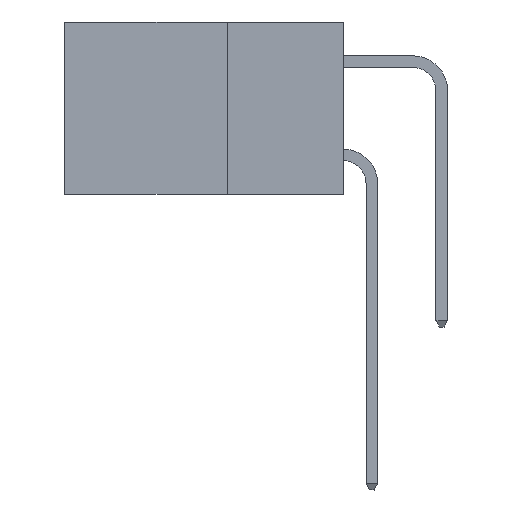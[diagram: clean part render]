
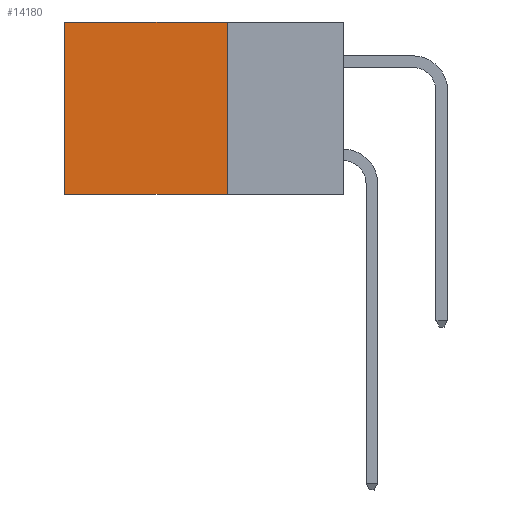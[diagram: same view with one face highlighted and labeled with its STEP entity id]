
A CAD part, left-side view. The second image highlights one B-rep face of the part: STEP entity #14180.
In plain terms, the highlighted planar face has unit normal (-1, 0, 0).
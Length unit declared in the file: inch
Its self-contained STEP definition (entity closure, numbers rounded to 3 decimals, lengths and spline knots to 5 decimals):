
#295 = ORIENTED_EDGE ( 'NONE', *, *, #18382, .F. ) ;
#797 = ORIENTED_EDGE ( 'NONE', *, *, #12884, .F. ) ;
#1860 = DIRECTION ( 'NONE',  ( 0., 1., 0. ) ) ;
#2047 = VECTOR ( 'NONE', #17260, 39.37008 ) ;
#2422 = CARTESIAN_POINT ( 'NONE',  ( 0.298, 0.25, 0. ) ) ;
#2615 = CARTESIAN_POINT ( 'NONE',  ( 0.298, 0.6, 0. ) ) ;
#2665 = VERTEX_POINT ( 'NONE', #2615 ) ;
#4156 = VECTOR ( 'NONE', #1860, 39.37008 ) ;
#5149 = CARTESIAN_POINT ( 'NONE',  ( 0.298, 0.6, 0. ) ) ;
#6287 = VECTOR ( 'NONE', #22823, 39.37008 ) ;
#6411 = CARTESIAN_POINT ( 'NONE',  ( 0.298, 0.25, -0.37 ) ) ;
#6612 = ORIENTED_EDGE ( 'NONE', *, *, #14780, .T. ) ;
#7228 = VERTEX_POINT ( 'NONE', #10940 ) ;
#8407 = CARTESIAN_POINT ( 'NONE',  ( 0.298, 0.6, -0.37 ) ) ;
#9844 = VECTOR ( 'NONE', #13920, 39.37008 ) ;
#9999 = DIRECTION ( 'NONE',  ( 0., 0., -1. ) ) ;
#10940 = CARTESIAN_POINT ( 'NONE',  ( 0.298, 0.25, 0. ) ) ;
#11346 = AXIS2_PLACEMENT_3D ( 'NONE', #20890, #17433, #9999 ) ;
#11804 = VERTEX_POINT ( 'NONE', #8407 ) ;
#11886 = LINE ( 'NONE', #5149, #9844 ) ;
#12165 = VERTEX_POINT ( 'NONE', #6411 ) ;
#12884 = EDGE_CURVE ( 'NONE', #12165, #11804, #23240, .T. ) ;
#13545 = ORIENTED_EDGE ( 'NONE', *, *, #16519, .T. ) ;
#13920 = DIRECTION ( 'NONE',  ( 0., 0., -1. ) ) ;
#14180 = ADVANCED_FACE ( 'NONE', ( #17979 ), #21041, .F. ) ;
#14780 = EDGE_CURVE ( 'NONE', #2665, #11804, #11886, .T. ) ;
#14796 = EDGE_LOOP ( 'NONE', ( #6612, #797, #295, #13545 ) ) ;
#14998 = CARTESIAN_POINT ( 'NONE',  ( 0.298, 0.25, -0.37 ) ) ;
#15563 = CARTESIAN_POINT ( 'NONE',  ( 0.298, 0.25, 0. ) ) ;
#16519 = EDGE_CURVE ( 'NONE', #7228, #2665, #18768, .T. ) ;
#17260 = DIRECTION ( 'NONE',  ( 0., 0., -1. ) ) ;
#17433 = DIRECTION ( 'NONE',  ( 1., 0., 0. ) ) ;
#17979 = FACE_OUTER_BOUND ( 'NONE', #14796, .T. ) ;
#18191 = LINE ( 'NONE', #15563, #2047 ) ;
#18382 = EDGE_CURVE ( 'NONE', #7228, #12165, #18191, .T. ) ;
#18768 = LINE ( 'NONE', #2422, #6287 ) ;
#20890 = CARTESIAN_POINT ( 'NONE',  ( 0.298, 0.25, 0. ) ) ;
#21041 = PLANE ( 'NONE',  #11346 ) ;
#22823 = DIRECTION ( 'NONE',  ( 0., 1., 0. ) ) ;
#23240 = LINE ( 'NONE', #14998, #4156 ) ;
